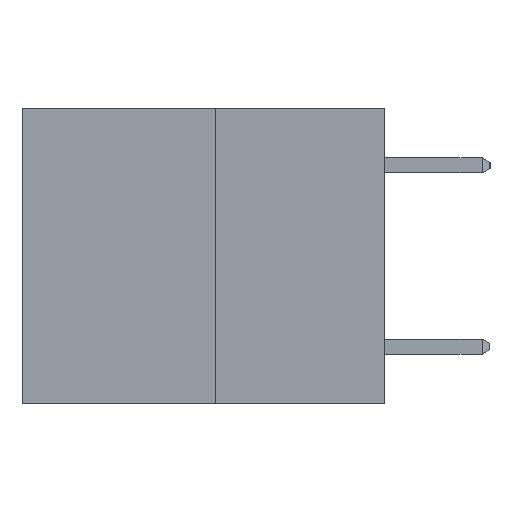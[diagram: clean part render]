
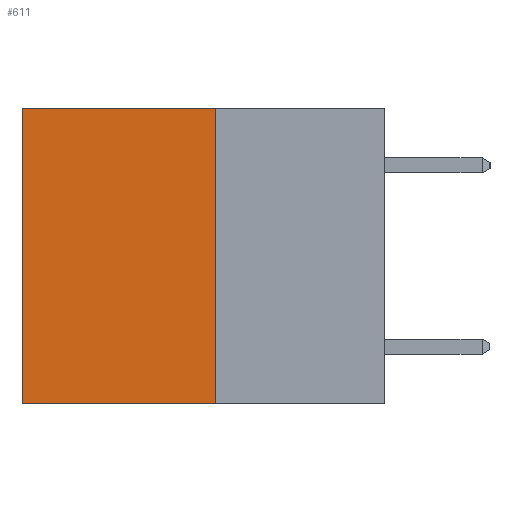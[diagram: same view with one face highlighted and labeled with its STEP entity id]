
A CAD part, left-side view. The second image highlights one B-rep face of the part: STEP entity #611.
In plain terms, the highlighted planar face has unit normal (-1, 0, 0).
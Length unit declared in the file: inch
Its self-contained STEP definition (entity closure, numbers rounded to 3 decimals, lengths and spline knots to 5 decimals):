
#611 = ADVANCED_FACE ( 'NONE', ( #11349 ), #6991, .F. ) ;
#896 = LINE ( 'NONE', #2838, #9139 ) ;
#1050 = DIRECTION ( 'NONE',  ( 0., 1., 0. ) ) ;
#1594 = VECTOR ( 'NONE', #1050, 39.37008 ) ;
#1595 = CARTESIAN_POINT ( 'NONE',  ( 0.3165, 0.28, -0.49 ) ) ;
#1905 = EDGE_CURVE ( 'NONE', #5798, #9327, #5238, .T. ) ;
#2311 = CARTESIAN_POINT ( 'NONE',  ( 0.3165, 0.28, -0.49 ) ) ;
#2838 = CARTESIAN_POINT ( 'NONE',  ( 0.3165, 0.6, -0.49 ) ) ;
#3239 = ORIENTED_EDGE ( 'NONE', *, *, #4678, .T. ) ;
#4209 = VECTOR ( 'NONE', #8007, 39.37008 ) ;
#4486 = LINE ( 'NONE', #10691, #4209 ) ;
#4538 = CARTESIAN_POINT ( 'NONE',  ( 0.3165, 0.28, -0.49 ) ) ;
#4678 = EDGE_CURVE ( 'NONE', #8375, #9327, #896, .T. ) ;
#4717 = DIRECTION ( 'NONE',  ( 0., 0., -1. ) ) ;
#5193 = VERTEX_POINT ( 'NONE', #10626 ) ;
#5238 = LINE ( 'NONE', #4538, #1594 ) ;
#5547 = DIRECTION ( 'NONE',  ( 0., 0., -1. ) ) ;
#5560 = EDGE_LOOP ( 'NONE', ( #3239, #7252, #10516, #10593 ) ) ;
#5798 = VERTEX_POINT ( 'NONE', #2311 ) ;
#6991 = PLANE ( 'NONE',  #10886 ) ;
#7196 = DIRECTION ( 'NONE',  ( 1., 0., 0. ) ) ;
#7252 = ORIENTED_EDGE ( 'NONE', *, *, #1905, .F. ) ;
#7386 = VECTOR ( 'NONE', #5547, 39.37008 ) ;
#7956 = LINE ( 'NONE', #9963, #7386 ) ;
#8007 = DIRECTION ( 'NONE',  ( 0., 1., 0. ) ) ;
#8036 = DIRECTION ( 'NONE',  ( 0., 0., -1. ) ) ;
#8375 = VERTEX_POINT ( 'NONE', #9193 ) ;
#8752 = CARTESIAN_POINT ( 'NONE',  ( 0.3165, 0.6, -0.49 ) ) ;
#9139 = VECTOR ( 'NONE', #4717, 39.37008 ) ;
#9193 = CARTESIAN_POINT ( 'NONE',  ( 0.3165, 0.6, 0. ) ) ;
#9299 = EDGE_CURVE ( 'NONE', #5193, #8375, #4486, .T. ) ;
#9327 = VERTEX_POINT ( 'NONE', #8752 ) ;
#9963 = CARTESIAN_POINT ( 'NONE',  ( 0.3165, 0.28, -0.49 ) ) ;
#10103 = EDGE_CURVE ( 'NONE', #5193, #5798, #7956, .T. ) ;
#10516 = ORIENTED_EDGE ( 'NONE', *, *, #10103, .F. ) ;
#10593 = ORIENTED_EDGE ( 'NONE', *, *, #9299, .T. ) ;
#10626 = CARTESIAN_POINT ( 'NONE',  ( 0.3165, 0.28, 0. ) ) ;
#10691 = CARTESIAN_POINT ( 'NONE',  ( 0.3165, 0.28, 0. ) ) ;
#10886 = AXIS2_PLACEMENT_3D ( 'NONE', #1595, #7196, #8036 ) ;
#11349 = FACE_OUTER_BOUND ( 'NONE', #5560, .T. ) ;
